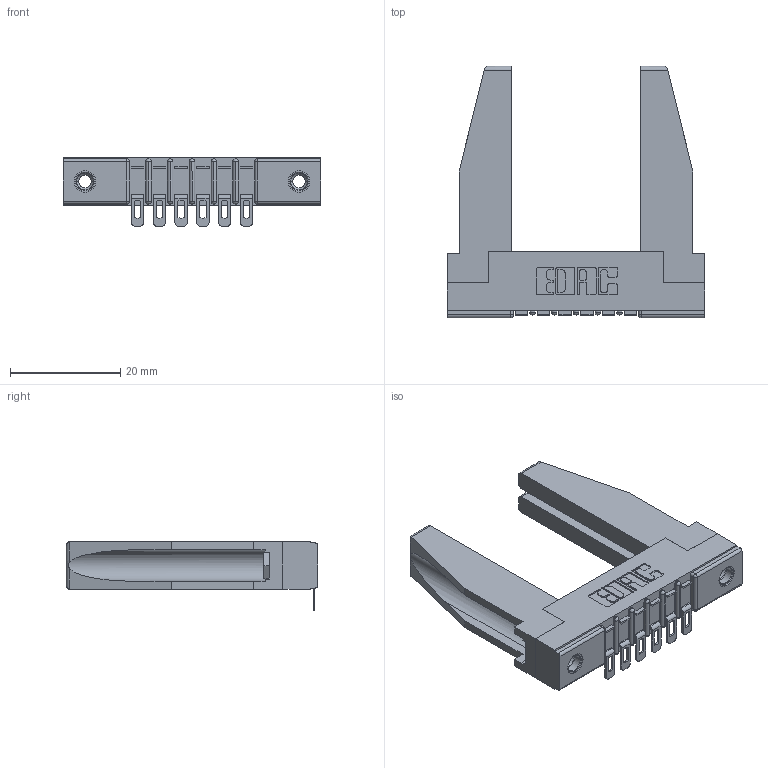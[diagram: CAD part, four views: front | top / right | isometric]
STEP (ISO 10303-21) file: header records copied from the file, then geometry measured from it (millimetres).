
FILE_DESCRIPTION (( 'STEP AP203' ), '1' );
FILE_NAME ('357-006-554-178.STEP', '2019-09-16T17:10:20', ( '' ), ( '' ), 'SwSTEP 2.0', 'SolidWorks 2016', '' );
FILE_SCHEMA (( 'CONFIG_CONTROL_DESIGN' ));
Length unit declared in the file: inch
Products named in the file (5): 357-006-554-178; 345-250-001_345-250-001-102; 307-290-002_554; 307-220-078; 307 Part_.156 Dia Mounting Holes
Assembly tree (11 placements, depth 2):
  357-006-554-178
    307 Part_.156 Dia Mounting Holes
    307-290-002_554  x6
    307-220-078  x2
    345-250-001_345-250-001-102  x2
Bounding box: 46.79 x 45.72 x 12.52 mm (x, y, z)
Volume: 7075.9 mm3; surface area: 8562.5 mm2
Topology: 11 solids, 11 shells, 741 faces, 2171 edges, 1418 vertices
Faces by surface type: plane 430, cylinder 281, sphere 14, cone 12, torus 4
Entity records: 12986 total; most frequent: CARTESIAN_POINT 2184, ORIENTED_EDGE 2130, DIRECTION 2101, EDGE_CURVE 1065, LINE 795, VECTOR 795, VERTEX_POINT 694, AXIS2_PLACEMENT_3D 653
